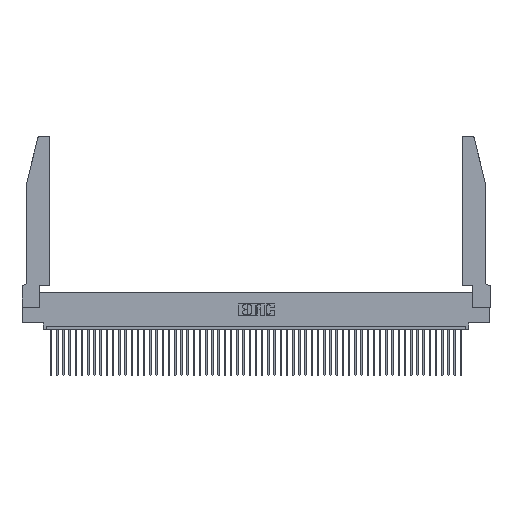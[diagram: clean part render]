
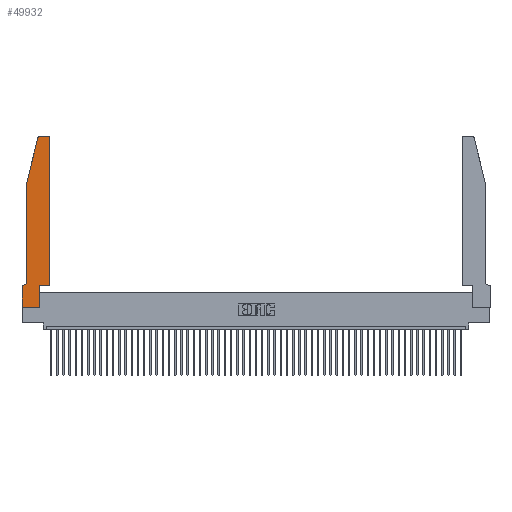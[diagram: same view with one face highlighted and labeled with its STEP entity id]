
A CAD part, top view. The second image highlights one B-rep face of the part: STEP entity #49932.
In plain terms, the highlighted planar face has unit normal (0, 0, 1).
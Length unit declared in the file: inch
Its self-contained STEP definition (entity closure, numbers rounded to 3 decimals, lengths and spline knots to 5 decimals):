
#856 = VECTOR ( 'NONE', #34684, 39.37008 ) ;
#2025 = LINE ( 'NONE', #42222, #34604 ) ;
#2304 = EDGE_CURVE ( 'NONE', #12974, #27570, #11449, .T. ) ;
#2988 = ORIENTED_EDGE ( 'NONE', *, *, #2304, .T. ) ;
#3401 = CARTESIAN_POINT ( 'NONE',  ( 0.0055, 0.42, 0.37 ) ) ;
#3420 = CARTESIAN_POINT ( 'NONE',  ( 0.284, 2.75, 0.37 ) ) ;
#3546 = CARTESIAN_POINT ( 'NONE',  ( 0.2605, 2.75, 0.37 ) ) ;
#3734 = EDGE_CURVE ( 'NONE', #46803, #7595, #26861, .T. ) ;
#4886 = CARTESIAN_POINT ( 'NONE',  ( 0.4505, 0.35, 0.37 ) ) ;
#5244 = EDGE_CURVE ( 'NONE', #27570, #46803, #50599, .T. ) ;
#5711 = LINE ( 'NONE', #31470, #37665 ) ;
#5894 = AXIS2_PLACEMENT_3D ( 'NONE', #13816, #17799, #11040 ) ;
#6781 = CARTESIAN_POINT ( 'NONE',  ( 0., 0., 0.37 ) ) ;
#6894 = CARTESIAN_POINT ( 'NONE',  ( 0.0755, 0.35, 0.37 ) ) ;
#6936 = EDGE_CURVE ( 'NONE', #13597, #41727, #50148, .T. ) ;
#7043 = DIRECTION ( 'NONE',  ( 0., 0., -1. ) ) ;
#7227 = LINE ( 'NONE', #6894, #856 ) ;
#7238 = CARTESIAN_POINT ( 'NONE',  ( 0., 0., 0.37 ) ) ;
#7476 = VECTOR ( 'NONE', #40027, 39.37008 ) ;
#7595 = VERTEX_POINT ( 'NONE', #47855 ) ;
#8861 = ORIENTED_EDGE ( 'NONE', *, *, #29168, .T. ) ;
#9254 = CARTESIAN_POINT ( 'NONE',  ( 0.284, 2.72, 0.37 ) ) ;
#11040 = DIRECTION ( 'NONE',  ( 1., 0., 0. ) ) ;
#11449 = LINE ( 'NONE', #24566, #51635 ) ;
#11890 = PLANE ( 'NONE',  #36967 ) ;
#12214 = DIRECTION ( 'NONE',  ( 0., 0., 1. ) ) ;
#12331 = EDGE_LOOP ( 'NONE', ( #44425, #36276, #8861, #17382, #12487, #14995, #39506, #32909, #22444, #2988, #28365, #37084 ) ) ;
#12487 = ORIENTED_EDGE ( 'NONE', *, *, #34642, .T. ) ;
#12524 = EDGE_CURVE ( 'NONE', #20341, #35738, #23235, .T. ) ;
#12947 = LINE ( 'NONE', #3546, #46930 ) ;
#12974 = VERTEX_POINT ( 'NONE', #26610 ) ;
#13597 = VERTEX_POINT ( 'NONE', #3420 ) ;
#13816 = CARTESIAN_POINT ( 'NONE',  ( 0.4205, 2.72, 0.37 ) ) ;
#14672 = CARTESIAN_POINT ( 'NONE',  ( 0.2865, 0., 0.37 ) ) ;
#14995 = ORIENTED_EDGE ( 'NONE', *, *, #44122, .T. ) ;
#15236 = CIRCLE ( 'NONE', #29400, 0.07 ) ;
#16879 = EDGE_CURVE ( 'NONE', #7595, #13597, #12947, .T. ) ;
#16980 = VECTOR ( 'NONE', #49650, 39.37008 ) ;
#17382 = ORIENTED_EDGE ( 'NONE', *, *, #29481, .T. ) ;
#17799 = DIRECTION ( 'NONE',  ( 0., 0., 1. ) ) ;
#18414 = VERTEX_POINT ( 'NONE', #32713 ) ;
#20092 = AXIS2_PLACEMENT_3D ( 'NONE', #9254, #39683, #33269 ) ;
#20341 = VERTEX_POINT ( 'NONE', #47592 ) ;
#21487 = CARTESIAN_POINT ( 'NONE',  ( 0.2865, 0.35, 0.37 ) ) ;
#22444 = ORIENTED_EDGE ( 'NONE', *, *, #47788, .T. ) ;
#23235 = LINE ( 'NONE', #7238, #34411 ) ;
#24099 = CARTESIAN_POINT ( 'NONE',  ( 0., 0.35, 0.37 ) ) ;
#24204 = CARTESIAN_POINT ( 'NONE',  ( 0.0755, 2., 0.37 ) ) ;
#24205 = CARTESIAN_POINT ( 'NONE',  ( 0., 0., 0.37 ) ) ;
#24394 = DIRECTION ( 'NONE',  ( 1., 0., 0. ) ) ;
#24511 = DIRECTION ( 'NONE',  ( 0., 1., 0. ) ) ;
#24566 = CARTESIAN_POINT ( 'NONE',  ( 0.4505, 0.35, 0.37 ) ) ;
#26610 = CARTESIAN_POINT ( 'NONE',  ( 0.2865, 0.35, 0.37 ) ) ;
#26817 = LINE ( 'NONE', #21487, #16980 ) ;
#26861 = CIRCLE ( 'NONE', #5894, 0.03 ) ;
#26874 = CARTESIAN_POINT ( 'NONE',  ( 0.4505, 0.35, 0.37 ) ) ;
#27570 = VERTEX_POINT ( 'NONE', #26874 ) ;
#28365 = ORIENTED_EDGE ( 'NONE', *, *, #5244, .T. ) ;
#29168 = EDGE_CURVE ( 'NONE', #41727, #29907, #2025, .T. ) ;
#29400 = AXIS2_PLACEMENT_3D ( 'NONE', #3401, #7043, #39459 ) ;
#29481 = EDGE_CURVE ( 'NONE', #29907, #18414, #5711, .T. ) ;
#29907 = VERTEX_POINT ( 'NONE', #24204 ) ;
#31470 = CARTESIAN_POINT ( 'NONE',  ( 0.0755, 2., 0.37 ) ) ;
#31555 = DIRECTION ( 'NONE',  ( 0., -1., 0. ) ) ;
#32149 = DIRECTION ( 'NONE',  ( 1., 0., 0. ) ) ;
#32713 = CARTESIAN_POINT ( 'NONE',  ( 0.0755, 0.42, 0.37 ) ) ;
#32909 = ORIENTED_EDGE ( 'NONE', *, *, #47642, .T. ) ;
#33269 = DIRECTION ( 'NONE',  ( 1., 0., 0. ) ) ;
#34411 = VECTOR ( 'NONE', #31555, 39.37008 ) ;
#34604 = VECTOR ( 'NONE', #45740, 39.37008 ) ;
#34642 = EDGE_CURVE ( 'NONE', #18414, #48849, #15236, .T. ) ;
#34684 = DIRECTION ( 'NONE',  ( -1., 0., 0. ) ) ;
#35738 = VERTEX_POINT ( 'NONE', #6781 ) ;
#36276 = ORIENTED_EDGE ( 'NONE', *, *, #6936, .T. ) ;
#36967 = AXIS2_PLACEMENT_3D ( 'NONE', #24099, #12214, #32149 ) ;
#37084 = ORIENTED_EDGE ( 'NONE', *, *, #3734, .T. ) ;
#37665 = VECTOR ( 'NONE', #40271, 39.37008 ) ;
#38273 = DIRECTION ( 'NONE',  ( -1., 0., 0. ) ) ;
#39459 = DIRECTION ( 'NONE',  ( -1., 0., 0. ) ) ;
#39506 = ORIENTED_EDGE ( 'NONE', *, *, #12524, .T. ) ;
#39683 = DIRECTION ( 'NONE',  ( 0., 0., 1. ) ) ;
#40027 = DIRECTION ( 'NONE',  ( 1., 0., 0. ) ) ;
#40271 = DIRECTION ( 'NONE',  ( 0., -1., 0. ) ) ;
#41727 = VERTEX_POINT ( 'NONE', #46844 ) ;
#42222 = CARTESIAN_POINT ( 'NONE',  ( 0.0755, 2., 0.37 ) ) ;
#43663 = CARTESIAN_POINT ( 'NONE',  ( 0.4505, 2.72, 0.37 ) ) ;
#44122 = EDGE_CURVE ( 'NONE', #48849, #20341, #7227, .T. ) ;
#44425 = ORIENTED_EDGE ( 'NONE', *, *, #16879, .T. ) ;
#44554 = CARTESIAN_POINT ( 'NONE',  ( 0.0055, 0.35, 0.37 ) ) ;
#45738 = LINE ( 'NONE', #24205, #7476 ) ;
#45740 = DIRECTION ( 'NONE',  ( -0.239, -0.971, 0. ) ) ;
#46709 = FACE_OUTER_BOUND ( 'NONE', #12331, .T. ) ;
#46803 = VERTEX_POINT ( 'NONE', #43663 ) ;
#46844 = CARTESIAN_POINT ( 'NONE',  ( 0.25487, 2.72718, 0.37 ) ) ;
#46930 = VECTOR ( 'NONE', #38273, 39.37008 ) ;
#47592 = CARTESIAN_POINT ( 'NONE',  ( 0., 0.35, 0.37 ) ) ;
#47642 = EDGE_CURVE ( 'NONE', #35738, #49681, #45738, .T. ) ;
#47788 = EDGE_CURVE ( 'NONE', #49681, #12974, #26817, .T. ) ;
#47855 = CARTESIAN_POINT ( 'NONE',  ( 0.4205, 2.75, 0.37 ) ) ;
#48849 = VERTEX_POINT ( 'NONE', #44554 ) ;
#49277 = VECTOR ( 'NONE', #24511, 39.37008 ) ;
#49650 = DIRECTION ( 'NONE',  ( 0., 1., 0. ) ) ;
#49681 = VERTEX_POINT ( 'NONE', #14672 ) ;
#49932 = ADVANCED_FACE ( 'NONE', ( #46709 ), #11890, .T. ) ;
#50148 = CIRCLE ( 'NONE', #20092, 0.03 ) ;
#50599 = LINE ( 'NONE', #4886, #49277 ) ;
#51635 = VECTOR ( 'NONE', #24394, 39.37008 ) ;
